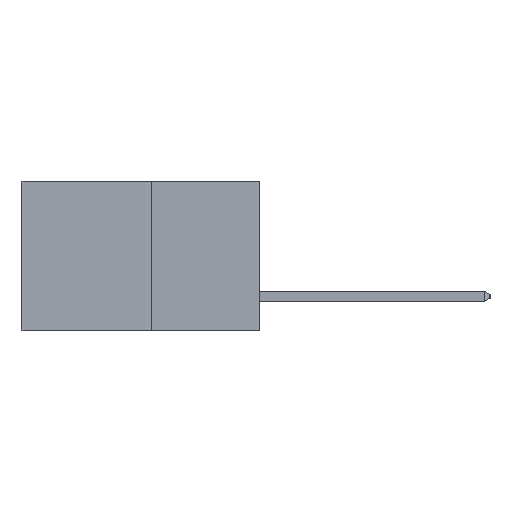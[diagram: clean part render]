
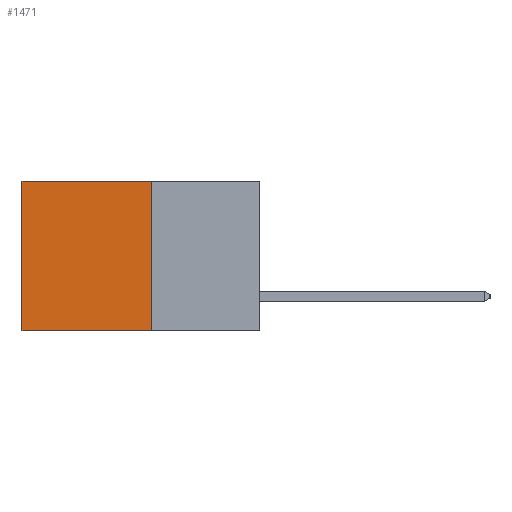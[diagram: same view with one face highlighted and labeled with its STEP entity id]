
A CAD part, left-side view. The second image highlights one B-rep face of the part: STEP entity #1471.
In plain terms, the highlighted planar face has unit normal (-1, 0, 0).
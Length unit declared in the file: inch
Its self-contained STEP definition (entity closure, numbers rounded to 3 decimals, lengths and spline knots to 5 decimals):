
#909 = ORIENTED_EDGE ( 'NONE', *, *, #11151, .T. ) ;
#994 = CARTESIAN_POINT ( 'NONE',  ( 0.277, 0.59, -0.37 ) ) ;
#1029 = CARTESIAN_POINT ( 'NONE',  ( 0.277, 0.59, 0. ) ) ;
#1186 = VERTEX_POINT ( 'NONE', #994 ) ;
#1471 = ADVANCED_FACE ( 'NONE', ( #2903 ), #19983, .F. ) ;
#2467 = VERTEX_POINT ( 'NONE', #1029 ) ;
#2903 = FACE_OUTER_BOUND ( 'NONE', #13531, .T. ) ;
#3696 = CARTESIAN_POINT ( 'NONE',  ( 0.277, 0.27, 0. ) ) ;
#5269 = ORIENTED_EDGE ( 'NONE', *, *, #7402, .F. ) ;
#5503 = CARTESIAN_POINT ( 'NONE',  ( 0.277, 0.27, -0.37 ) ) ;
#5750 = DIRECTION ( 'NONE',  ( 1., 0., 0. ) ) ;
#6687 = ORIENTED_EDGE ( 'NONE', *, *, #25263, .F. ) ;
#6708 = AXIS2_PLACEMENT_3D ( 'NONE', #5503, #5750, #11583 ) ;
#7402 = EDGE_CURVE ( 'NONE', #16874, #8555, #12779, .T. ) ;
#8555 = VERTEX_POINT ( 'NONE', #26613 ) ;
#9334 = LINE ( 'NONE', #21371, #20366 ) ;
#10466 = DIRECTION ( 'NONE',  ( 0., 1., 0. ) ) ;
#10838 = DIRECTION ( 'NONE',  ( 0., 0., -1. ) ) ;
#10863 = DIRECTION ( 'NONE',  ( 0., 0., -1. ) ) ;
#11151 = EDGE_CURVE ( 'NONE', #16874, #2467, #18261, .T. ) ;
#11583 = DIRECTION ( 'NONE',  ( 0., 0., -1. ) ) ;
#12514 = EDGE_CURVE ( 'NONE', #2467, #1186, #20845, .T. ) ;
#12779 = LINE ( 'NONE', #23207, #23767 ) ;
#13531 = EDGE_LOOP ( 'NONE', ( #16287, #6687, #5269, #909 ) ) ;
#15325 = VECTOR ( 'NONE', #10863, 39.37008 ) ;
#16287 = ORIENTED_EDGE ( 'NONE', *, *, #12514, .T. ) ;
#16874 = VERTEX_POINT ( 'NONE', #3696 ) ;
#16922 = CARTESIAN_POINT ( 'NONE',  ( 0.277, 0.59, -0.37 ) ) ;
#18261 = LINE ( 'NONE', #20804, #23101 ) ;
#19983 = PLANE ( 'NONE',  #6708 ) ;
#20366 = VECTOR ( 'NONE', #23321, 39.37008 ) ;
#20804 = CARTESIAN_POINT ( 'NONE',  ( 0.277, 0.27, 0. ) ) ;
#20845 = LINE ( 'NONE', #16922, #15325 ) ;
#21371 = CARTESIAN_POINT ( 'NONE',  ( 0.277, 0.27, -0.37 ) ) ;
#23101 = VECTOR ( 'NONE', #10466, 39.37008 ) ;
#23207 = CARTESIAN_POINT ( 'NONE',  ( 0.277, 0.27, -0.37 ) ) ;
#23321 = DIRECTION ( 'NONE',  ( 0., 1., 0. ) ) ;
#23767 = VECTOR ( 'NONE', #10838, 39.37008 ) ;
#25263 = EDGE_CURVE ( 'NONE', #8555, #1186, #9334, .T. ) ;
#26613 = CARTESIAN_POINT ( 'NONE',  ( 0.277, 0.27, -0.37 ) ) ;
